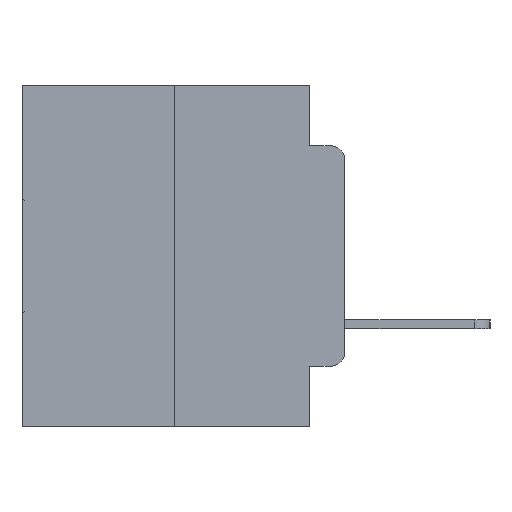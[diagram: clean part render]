
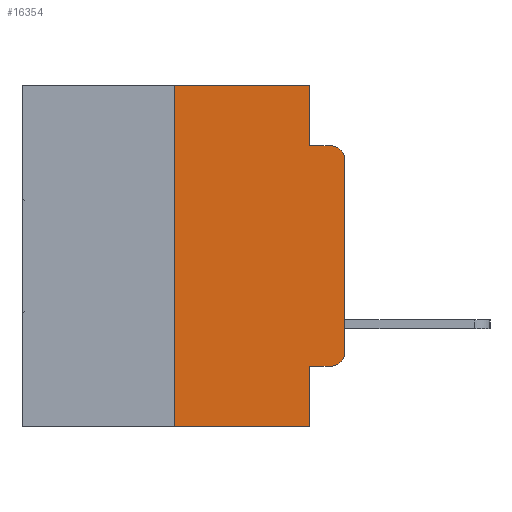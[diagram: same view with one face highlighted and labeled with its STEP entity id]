
A CAD part, left-side view. The second image highlights one B-rep face of the part: STEP entity #16354.
In plain terms, the highlighted planar face has unit normal (-1, 0, 0).
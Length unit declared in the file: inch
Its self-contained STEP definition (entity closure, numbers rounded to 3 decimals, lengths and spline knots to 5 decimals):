
#1277 = EDGE_LOOP ( 'NONE', ( #23757, #21374, #23257, #23416, #5322, #15748, #18978, #24774, #15271, #23131 ) ) ;
#1293 = VECTOR ( 'NONE', #17777, 39.37008 ) ;
#1418 = FACE_OUTER_BOUND ( 'NONE', #1277, .T. ) ;
#1721 = EDGE_CURVE ( 'NONE', #16682, #25502, #3744, .T. ) ;
#2207 = AXIS2_PLACEMENT_3D ( 'NONE', #21731, #8435, #23952 ) ;
#3138 = VERTEX_POINT ( 'NONE', #8507 ) ;
#3294 = LINE ( 'NONE', #22490, #20506 ) ;
#3721 = VERTEX_POINT ( 'NONE', #21590 ) ;
#3744 = LINE ( 'NONE', #22149, #26777 ) ;
#4055 = EDGE_CURVE ( 'NONE', #12394, #3138, #3294, .T. ) ;
#4109 = CARTESIAN_POINT ( 'NONE',  ( 0., 0.473, -0.5 ) ) ;
#4236 = VECTOR ( 'NONE', #21442, 39.37008 ) ;
#5015 = DIRECTION ( 'NONE',  ( 0., -1., 0. ) ) ;
#5090 = EDGE_CURVE ( 'NONE', #6677, #12394, #23570, .T. ) ;
#5322 = ORIENTED_EDGE ( 'NONE', *, *, #4055, .F. ) ;
#6677 = VERTEX_POINT ( 'NONE', #24382 ) ;
#7531 = LINE ( 'NONE', #18834, #1293 ) ;
#7827 = VERTEX_POINT ( 'NONE', #11089 ) ;
#8076 = CARTESIAN_POINT ( 'NONE',  ( 0., 0., -0.1085 ) ) ;
#8150 = EDGE_CURVE ( 'NONE', #3721, #13410, #25365, .T. ) ;
#8435 = DIRECTION ( 'NONE',  ( -1., 0., 0. ) ) ;
#8507 = CARTESIAN_POINT ( 'NONE',  ( 0., 0.051, 0. ) ) ;
#8515 = VERTEX_POINT ( 'NONE', #9001 ) ;
#9001 = CARTESIAN_POINT ( 'NONE',  ( 0., 0.051, -0.4115 ) ) ;
#9904 = CARTESIAN_POINT ( 'NONE',  ( 0., 0.051, -0.0885 ) ) ;
#11089 = CARTESIAN_POINT ( 'NONE',  ( 0., 0.02, -0.4115 ) ) ;
#11160 = EDGE_CURVE ( 'NONE', #25502, #13410, #21416, .T. ) ;
#11832 = CARTESIAN_POINT ( 'NONE',  ( 0., 0.25, 0. ) ) ;
#11870 = DIRECTION ( 'NONE',  ( -1., 0., 0. ) ) ;
#12394 = VERTEX_POINT ( 'NONE', #11832 ) ;
#12646 = EDGE_CURVE ( 'NONE', #8515, #7827, #27888, .T. ) ;
#12681 = CARTESIAN_POINT ( 'NONE',  ( 0., 0.051, -0.4115 ) ) ;
#13410 = VERTEX_POINT ( 'NONE', #29010 ) ;
#13623 = VECTOR ( 'NONE', #18844, 39.37008 ) ;
#14820 = VECTOR ( 'NONE', #15316, 39.37008 ) ;
#15271 = ORIENTED_EDGE ( 'NONE', *, *, #12646, .T. ) ;
#15316 = DIRECTION ( 'NONE',  ( 0., -1., 0. ) ) ;
#15748 = ORIENTED_EDGE ( 'NONE', *, *, #5090, .F. ) ;
#15751 = DIRECTION ( 'NONE',  ( 0., 0., -1. ) ) ;
#16223 = VERTEX_POINT ( 'NONE', #28382 ) ;
#16354 = ADVANCED_FACE ( 'NONE', ( #1418 ), #28936, .F. ) ;
#16682 = VERTEX_POINT ( 'NONE', #23594 ) ;
#17777 = DIRECTION ( 'NONE',  ( 0., 0., -1. ) ) ;
#18834 = CARTESIAN_POINT ( 'NONE',  ( 0., 0.051, 0. ) ) ;
#18844 = DIRECTION ( 'NONE',  ( 0., -1., 0. ) ) ;
#18978 = ORIENTED_EDGE ( 'NONE', *, *, #27022, .T. ) ;
#19330 = AXIS2_PLACEMENT_3D ( 'NONE', #26753, #22338, #15751 ) ;
#20172 = CARTESIAN_POINT ( 'NONE',  ( 0., 0.25, 0. ) ) ;
#20252 = DIRECTION ( 'NONE',  ( 0., 0., 1. ) ) ;
#20506 = VECTOR ( 'NONE', #5015, 39.37008 ) ;
#21374 = ORIENTED_EDGE ( 'NONE', *, *, #11160, .T. ) ;
#21416 = CIRCLE ( 'NONE', #27858, 0.02 ) ;
#21420 = LINE ( 'NONE', #4109, #14820 ) ;
#21442 = DIRECTION ( 'NONE',  ( 0., 0., -1. ) ) ;
#21553 = EDGE_CURVE ( 'NONE', #7827, #16682, #23673, .T. ) ;
#21590 = CARTESIAN_POINT ( 'NONE',  ( 0., 0.051, -0.0885 ) ) ;
#21647 = DIRECTION ( 'NONE',  ( 0., 0., 1. ) ) ;
#21731 = CARTESIAN_POINT ( 'NONE',  ( 0., 0.02, -0.3915 ) ) ;
#22052 = VECTOR ( 'NONE', #28113, 39.37008 ) ;
#22149 = CARTESIAN_POINT ( 'NONE',  ( 0., 0., 0. ) ) ;
#22338 = DIRECTION ( 'NONE',  ( 1., 0., 0. ) ) ;
#22490 = CARTESIAN_POINT ( 'NONE',  ( 0., 0.473, 0. ) ) ;
#22809 = LINE ( 'NONE', #23670, #4236 ) ;
#22869 = VECTOR ( 'NONE', #20252, 39.37008 ) ;
#23131 = ORIENTED_EDGE ( 'NONE', *, *, #21553, .T. ) ;
#23257 = ORIENTED_EDGE ( 'NONE', *, *, #8150, .F. ) ;
#23416 = ORIENTED_EDGE ( 'NONE', *, *, #24503, .F. ) ;
#23570 = LINE ( 'NONE', #20172, #22869 ) ;
#23594 = CARTESIAN_POINT ( 'NONE',  ( 0., 0., -0.3915 ) ) ;
#23670 = CARTESIAN_POINT ( 'NONE',  ( 0., 0.051, 0. ) ) ;
#23673 = CIRCLE ( 'NONE', #2207, 0.02 ) ;
#23757 = ORIENTED_EDGE ( 'NONE', *, *, #1721, .T. ) ;
#23952 = DIRECTION ( 'NONE',  ( 0., 0., -1. ) ) ;
#24382 = CARTESIAN_POINT ( 'NONE',  ( 0., 0.25, -0.5 ) ) ;
#24503 = EDGE_CURVE ( 'NONE', #3138, #3721, #7531, .T. ) ;
#24774 = ORIENTED_EDGE ( 'NONE', *, *, #28880, .F. ) ;
#25082 = CARTESIAN_POINT ( 'NONE',  ( 0., 0.02, -0.1085 ) ) ;
#25365 = LINE ( 'NONE', #9904, #13623 ) ;
#25502 = VERTEX_POINT ( 'NONE', #8076 ) ;
#26753 = CARTESIAN_POINT ( 'NONE',  ( 0., 0.473, 0. ) ) ;
#26777 = VECTOR ( 'NONE', #21647, 39.37008 ) ;
#27022 = EDGE_CURVE ( 'NONE', #6677, #16223, #21420, .T. ) ;
#27300 = DIRECTION ( 'NONE',  ( 0., 0., -1. ) ) ;
#27858 = AXIS2_PLACEMENT_3D ( 'NONE', #25082, #11870, #27300 ) ;
#27888 = LINE ( 'NONE', #12681, #22052 ) ;
#28113 = DIRECTION ( 'NONE',  ( 0., -1., 0. ) ) ;
#28382 = CARTESIAN_POINT ( 'NONE',  ( 0., 0.051, -0.5 ) ) ;
#28880 = EDGE_CURVE ( 'NONE', #8515, #16223, #22809, .T. ) ;
#28936 = PLANE ( 'NONE',  #19330 ) ;
#29010 = CARTESIAN_POINT ( 'NONE',  ( 0., 0.02, -0.0885 ) ) ;
